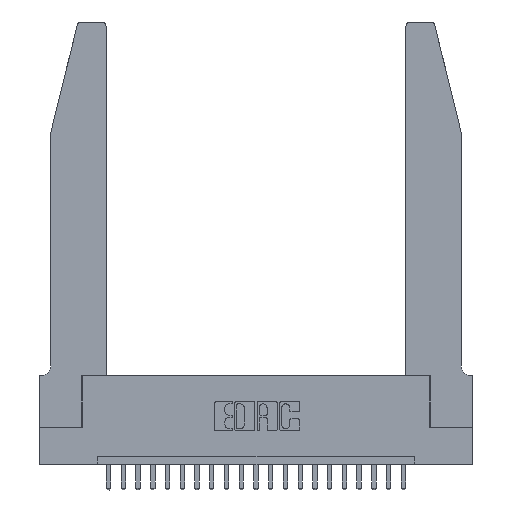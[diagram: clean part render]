
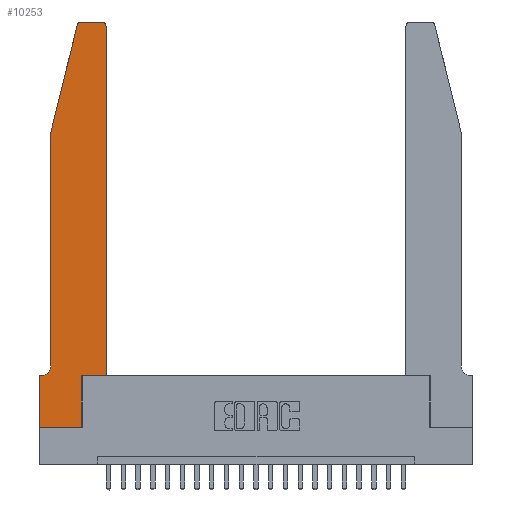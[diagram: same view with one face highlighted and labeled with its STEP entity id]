
A CAD part, top view. The second image highlights one B-rep face of the part: STEP entity #10253.
In plain terms, the highlighted planar face has unit normal (0, 0, 1).
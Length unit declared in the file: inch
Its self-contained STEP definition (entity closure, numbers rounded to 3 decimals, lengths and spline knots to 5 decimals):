
#372 = CARTESIAN_POINT ( 'NONE',  ( 0.0755, 2., 0.37 ) ) ;
#571 = VERTEX_POINT ( 'NONE', #3182 ) ;
#725 = DIRECTION ( 'NONE',  ( 0., 1., 0. ) ) ;
#789 = CARTESIAN_POINT ( 'NONE',  ( 0., 0., 0.37 ) ) ;
#870 = CIRCLE ( 'NONE', #2575, 0.03 ) ;
#1457 = CARTESIAN_POINT ( 'NONE',  ( 0.4205, 2.72, 0.37 ) ) ;
#1518 = CARTESIAN_POINT ( 'NONE',  ( 0.4505, 0.35, 0.37 ) ) ;
#1692 = DIRECTION ( 'NONE',  ( 0., 1., 0. ) ) ;
#2137 = DIRECTION ( 'NONE',  ( 0., -1., 0. ) ) ;
#2445 = CARTESIAN_POINT ( 'NONE',  ( 0.0755, 2., 0.37 ) ) ;
#2463 = VECTOR ( 'NONE', #1692, 39.37008 ) ;
#2575 = AXIS2_PLACEMENT_3D ( 'NONE', #1457, #5123, #5195 ) ;
#2932 = DIRECTION ( 'NONE',  ( 0., -1., 0. ) ) ;
#3182 = CARTESIAN_POINT ( 'NONE',  ( 0.4505, 0.35, 0.37 ) ) ;
#4359 = VECTOR ( 'NONE', #18273, 39.37008 ) ;
#4439 = LINE ( 'NONE', #1518, #2463 ) ;
#4451 = ORIENTED_EDGE ( 'NONE', *, *, #13753, .T. ) ;
#5123 = DIRECTION ( 'NONE',  ( 0., 0., 1. ) ) ;
#5195 = DIRECTION ( 'NONE',  ( 1., 0., 0. ) ) ;
#5236 = EDGE_CURVE ( 'NONE', #571, #22540, #4439, .T. ) ;
#5314 = CARTESIAN_POINT ( 'NONE',  ( 0.284, 2.72, 0.37 ) ) ;
#5346 = VERTEX_POINT ( 'NONE', #18150 ) ;
#5391 = PLANE ( 'NONE',  #16368 ) ;
#5897 = FACE_OUTER_BOUND ( 'NONE', #10916, .T. ) ;
#5898 = EDGE_CURVE ( 'NONE', #15645, #22843, #13520, .T. ) ;
#6020 = CARTESIAN_POINT ( 'NONE',  ( 0.4505, 0.35, 0.37 ) ) ;
#6028 = CARTESIAN_POINT ( 'NONE',  ( 0.25487, 2.72718, 0.37 ) ) ;
#6713 = CARTESIAN_POINT ( 'NONE',  ( 0.284, 2.75, 0.37 ) ) ;
#7237 = DIRECTION ( 'NONE',  ( 0., 0., 1. ) ) ;
#7592 = VECTOR ( 'NONE', #22537, 39.37008 ) ;
#7666 = EDGE_CURVE ( 'NONE', #15304, #571, #8349, .T. ) ;
#7699 = CARTESIAN_POINT ( 'NONE',  ( 0.0055, 0.35, 0.37 ) ) ;
#8037 = EDGE_CURVE ( 'NONE', #12215, #15304, #15685, .T. ) ;
#8349 = LINE ( 'NONE', #6020, #4359 ) ;
#8727 = VECTOR ( 'NONE', #10190, 39.37008 ) ;
#8914 = CARTESIAN_POINT ( 'NONE',  ( 0.4505, 2.72, 0.37 ) ) ;
#9257 = CIRCLE ( 'NONE', #21965, 0.03 ) ;
#10008 = ORIENTED_EDGE ( 'NONE', *, *, #19811, .T. ) ;
#10104 = VECTOR ( 'NONE', #2932, 39.37008 ) ;
#10190 = DIRECTION ( 'NONE',  ( -0.239, -0.971, 0. ) ) ;
#10253 = ADVANCED_FACE ( 'NONE', ( #5897 ), #5391, .T. ) ;
#10676 = ORIENTED_EDGE ( 'NONE', *, *, #17089, .T. ) ;
#10916 = EDGE_LOOP ( 'NONE', ( #10676, #15373, #11937, #17128, #20375, #20714, #10008, #12366, #19722, #15523, #21319, #4451 ) ) ;
#11093 = LINE ( 'NONE', #789, #14785 ) ;
#11251 = EDGE_CURVE ( 'NONE', #23357, #15295, #13508, .T. ) ;
#11601 = CARTESIAN_POINT ( 'NONE',  ( 0.2865, 0.35, 0.37 ) ) ;
#11937 = ORIENTED_EDGE ( 'NONE', *, *, #5898, .T. ) ;
#12088 = VERTEX_POINT ( 'NONE', #6713 ) ;
#12118 = DIRECTION ( 'NONE',  ( -1., 0., 0. ) ) ;
#12215 = VERTEX_POINT ( 'NONE', #16318 ) ;
#12290 = VECTOR ( 'NONE', #2137, 39.37008 ) ;
#12366 = ORIENTED_EDGE ( 'NONE', *, *, #14973, .T. ) ;
#13169 = LINE ( 'NONE', #372, #12290 ) ;
#13310 = LINE ( 'NONE', #21382, #20697 ) ;
#13508 = LINE ( 'NONE', #15163, #7592 ) ;
#13520 = LINE ( 'NONE', #22397, #8727 ) ;
#13753 = EDGE_CURVE ( 'NONE', #22540, #19236, #870, .T. ) ;
#13913 = CARTESIAN_POINT ( 'NONE',  ( 0.4205, 2.75, 0.37 ) ) ;
#14444 = CARTESIAN_POINT ( 'NONE',  ( 0., 0.35, 0.37 ) ) ;
#14599 = DIRECTION ( 'NONE',  ( 1., 0., 0. ) ) ;
#14785 = VECTOR ( 'NONE', #15250, 39.37008 ) ;
#14973 = EDGE_CURVE ( 'NONE', #5346, #12215, #11093, .T. ) ;
#15163 = CARTESIAN_POINT ( 'NONE',  ( 0.0755, 0.35, 0.37 ) ) ;
#15250 = DIRECTION ( 'NONE',  ( 1., 0., 0. ) ) ;
#15295 = VERTEX_POINT ( 'NONE', #14444 ) ;
#15304 = VERTEX_POINT ( 'NONE', #19923 ) ;
#15328 = EDGE_CURVE ( 'NONE', #12088, #15645, #9257, .T. ) ;
#15373 = ORIENTED_EDGE ( 'NONE', *, *, #15328, .T. ) ;
#15523 = ORIENTED_EDGE ( 'NONE', *, *, #7666, .T. ) ;
#15645 = VERTEX_POINT ( 'NONE', #6028 ) ;
#15685 = LINE ( 'NONE', #11601, #19110 ) ;
#15872 = DIRECTION ( 'NONE',  ( 0., 0., -1. ) ) ;
#16052 = LINE ( 'NONE', #20731, #10104 ) ;
#16230 = DIRECTION ( 'NONE',  ( -1., 0., 0. ) ) ;
#16318 = CARTESIAN_POINT ( 'NONE',  ( 0.2865, 0., 0.37 ) ) ;
#16368 = AXIS2_PLACEMENT_3D ( 'NONE', #17965, #19754, #19919 ) ;
#17089 = EDGE_CURVE ( 'NONE', #19236, #12088, #13310, .T. ) ;
#17128 = ORIENTED_EDGE ( 'NONE', *, *, #20238, .T. ) ;
#17225 = CIRCLE ( 'NONE', #17622, 0.07 ) ;
#17622 = AXIS2_PLACEMENT_3D ( 'NONE', #21274, #15872, #12118 ) ;
#17965 = CARTESIAN_POINT ( 'NONE',  ( 0., 0.35, 0.37 ) ) ;
#18150 = CARTESIAN_POINT ( 'NONE',  ( 0., 0., 0.37 ) ) ;
#18273 = DIRECTION ( 'NONE',  ( 1., 0., 0. ) ) ;
#19110 = VECTOR ( 'NONE', #725, 39.37008 ) ;
#19236 = VERTEX_POINT ( 'NONE', #13913 ) ;
#19722 = ORIENTED_EDGE ( 'NONE', *, *, #8037, .T. ) ;
#19754 = DIRECTION ( 'NONE',  ( 0., 0., 1. ) ) ;
#19811 = EDGE_CURVE ( 'NONE', #15295, #5346, #16052, .T. ) ;
#19849 = EDGE_CURVE ( 'NONE', #22863, #23357, #17225, .T. ) ;
#19919 = DIRECTION ( 'NONE',  ( 1., 0., 0. ) ) ;
#19923 = CARTESIAN_POINT ( 'NONE',  ( 0.2865, 0.35, 0.37 ) ) ;
#20238 = EDGE_CURVE ( 'NONE', #22843, #22863, #13169, .T. ) ;
#20375 = ORIENTED_EDGE ( 'NONE', *, *, #19849, .T. ) ;
#20690 = CARTESIAN_POINT ( 'NONE',  ( 0.0755, 0.42, 0.37 ) ) ;
#20697 = VECTOR ( 'NONE', #16230, 39.37008 ) ;
#20714 = ORIENTED_EDGE ( 'NONE', *, *, #11251, .T. ) ;
#20731 = CARTESIAN_POINT ( 'NONE',  ( 0., 0., 0.37 ) ) ;
#21274 = CARTESIAN_POINT ( 'NONE',  ( 0.0055, 0.42, 0.37 ) ) ;
#21319 = ORIENTED_EDGE ( 'NONE', *, *, #5236, .T. ) ;
#21382 = CARTESIAN_POINT ( 'NONE',  ( 0.2605, 2.75, 0.37 ) ) ;
#21965 = AXIS2_PLACEMENT_3D ( 'NONE', #5314, #7237, #14599 ) ;
#22397 = CARTESIAN_POINT ( 'NONE',  ( 0.0755, 2., 0.37 ) ) ;
#22537 = DIRECTION ( 'NONE',  ( -1., 0., 0. ) ) ;
#22540 = VERTEX_POINT ( 'NONE', #8914 ) ;
#22843 = VERTEX_POINT ( 'NONE', #2445 ) ;
#22863 = VERTEX_POINT ( 'NONE', #20690 ) ;
#23357 = VERTEX_POINT ( 'NONE', #7699 ) ;
